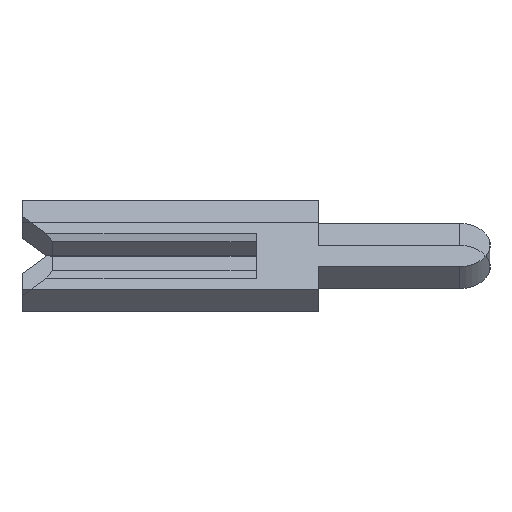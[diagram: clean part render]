
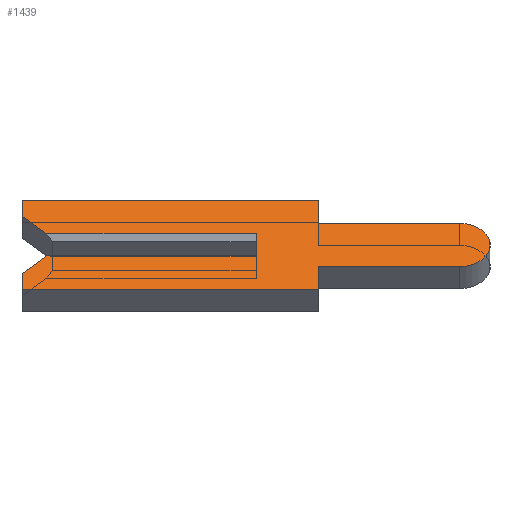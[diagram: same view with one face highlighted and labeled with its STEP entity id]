
A CAD part, left-side view. The second image highlights one B-rep face of the part: STEP entity #1439.
In plain terms, the highlighted face is planar.
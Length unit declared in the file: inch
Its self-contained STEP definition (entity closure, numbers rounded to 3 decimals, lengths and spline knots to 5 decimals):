
#7 = DIRECTION ( 'NONE',  ( 0., -1., 0. ) ) ;
#17 = DIRECTION ( 'NONE',  ( 0., 0., -1. ) ) ;
#46 = VERTEX_POINT ( 'NONE', #1941 ) ;
#65 = LINE ( 'NONE', #826, #1199 ) ;
#94 = VERTEX_POINT ( 'NONE', #2145 ) ;
#114 = EDGE_CURVE ( 'NONE', #2281, #2518, #854, .T. ) ;
#122 = CARTESIAN_POINT ( 'NONE',  ( -0.01, -0.04, 0.0195 ) ) ;
#156 = CARTESIAN_POINT ( 'NONE',  ( -0.01, 0.15, 0.026 ) ) ;
#189 = CARTESIAN_POINT ( 'NONE',  ( -0.01, -0.1305, 0.0195 ) ) ;
#202 = VERTEX_POINT ( 'NONE', #189 ) ;
#210 = VECTOR ( 'NONE', #1328, 39.37008 ) ;
#230 = EDGE_CURVE ( 'NONE', #1036, #2063, #1580, .T. ) ;
#243 = LINE ( 'NONE', #156, #2073 ) ;
#271 = EDGE_CURVE ( 'NONE', #1648, #94, #506, .T. ) ;
#272 = VECTOR ( 'NONE', #17, 39.37008 ) ;
#276 = VECTOR ( 'NONE', #582, 39.37008 ) ;
#277 = LINE ( 'NONE', #926, #210 ) ;
#283 = CARTESIAN_POINT ( 'NONE',  ( -0.01, 0.134, 0.01 ) ) ;
#305 = PLANE ( 'NONE',  #306 ) ;
#306 = AXIS2_PLACEMENT_3D ( 'NONE', #1707, #718, #921 ) ;
#350 = CARTESIAN_POINT ( 'NONE',  ( -0.01, 0.15, -0.04 ) ) ;
#405 = FACE_OUTER_BOUND ( 'NONE', #1035, .T. ) ;
#424 = EDGE_CURVE ( 'NONE', #1326, #1935, #1843, .T. ) ;
#500 = VECTOR ( 'NONE', #2418, 39.37008 ) ;
#506 = LINE ( 'NONE', #614, #1052 ) ;
#560 = VECTOR ( 'NONE', #1524, 39.37008 ) ;
#563 = DIRECTION ( 'NONE',  ( 0., 1., 0. ) ) ;
#579 = CARTESIAN_POINT ( 'NONE',  ( -0.01, 0.134, -0.01 ) ) ;
#582 = DIRECTION ( 'NONE',  ( 0., -0.707, 0.707 ) ) ;
#612 = VERTEX_POINT ( 'NONE', #2058 ) ;
#614 = CARTESIAN_POINT ( 'NONE',  ( -0.01, 0.15, 0.04 ) ) ;
#648 = EDGE_CURVE ( 'NONE', #202, #1647, #860, .T. ) ;
#718 = DIRECTION ( 'NONE',  ( 1., 0., 0. ) ) ;
#787 = VECTOR ( 'NONE', #2552, 39.37008 ) ;
#804 = CARTESIAN_POINT ( 'NONE',  ( -0.01, 0.1305, 0.0065 ) ) ;
#819 = VECTOR ( 'NONE', #1531, 39.37008 ) ;
#826 = CARTESIAN_POINT ( 'NONE',  ( -0.01, 0.15, 0.01 ) ) ;
#829 = ORIENTED_EDGE ( 'NONE', *, *, #1122, .F. ) ;
#854 = LINE ( 'NONE', #1562, #276 ) ;
#860 = CIRCLE ( 'NONE', #1827, 0.0195 ) ;
#907 = ORIENTED_EDGE ( 'NONE', *, *, #2233, .F. ) ;
#910 = CARTESIAN_POINT ( 'NONE',  ( -0.01, -0.04, -0.0195 ) ) ;
#921 = DIRECTION ( 'NONE',  ( 0., 0., -1. ) ) ;
#926 = CARTESIAN_POINT ( 'NONE',  ( -0.01, 0.15, -0.026 ) ) ;
#945 = LINE ( 'NONE', #1614, #1886 ) ;
#969 = CARTESIAN_POINT ( 'NONE',  ( -0.01, 0.15, 0.04 ) ) ;
#1035 = EDGE_LOOP ( 'NONE', ( #1040, #829, #907, #2174, #1686, #1324, #2101, #2035, #1656, #2122, #1872, #2027, #1849, #1943 ) ) ;
#1036 = VERTEX_POINT ( 'NONE', #283 ) ;
#1040 = ORIENTED_EDGE ( 'NONE', *, *, #2375, .T. ) ;
#1052 = VECTOR ( 'NONE', #1826, 39.37008 ) ;
#1113 = CARTESIAN_POINT ( 'NONE',  ( -0.01, 0., 0.0065 ) ) ;
#1122 = EDGE_CURVE ( 'NONE', #2093, #46, #1205, .T. ) ;
#1175 = EDGE_CURVE ( 'NONE', #612, #202, #1953, .T. ) ;
#1193 = EDGE_CURVE ( 'NONE', #1728, #2281, #277, .T. ) ;
#1199 = VECTOR ( 'NONE', #7, 39.37008 ) ;
#1205 = LINE ( 'NONE', #1113, #787 ) ;
#1277 = VECTOR ( 'NONE', #563, 39.37008 ) ;
#1319 = CARTESIAN_POINT ( 'NONE',  ( -0.01, -0.1305, 0. ) ) ;
#1324 = ORIENTED_EDGE ( 'NONE', *, *, #2412, .F. ) ;
#1326 = VERTEX_POINT ( 'NONE', #910 ) ;
#1328 = DIRECTION ( 'NONE',  ( 0., 0., 1. ) ) ;
#1382 = EDGE_CURVE ( 'NONE', #94, #612, #2306, .T. ) ;
#1439 = ADVANCED_FACE ( 'NONE', ( #405 ), #305, .F. ) ;
#1490 = LINE ( 'NONE', #2156, #1277 ) ;
#1524 = DIRECTION ( 'NONE',  ( 0., 0., -1. ) ) ;
#1531 = DIRECTION ( 'NONE',  ( 0., -1., 0. ) ) ;
#1562 = CARTESIAN_POINT ( 'NONE',  ( -0.01, 0.1305, -0.0065 ) ) ;
#1566 = CARTESIAN_POINT ( 'NONE',  ( -0.01, 0.15, 0.026 ) ) ;
#1580 = LINE ( 'NONE', #804, #500 ) ;
#1614 = CARTESIAN_POINT ( 'NONE',  ( -0.01, -0.1305, -0.01 ) ) ;
#1647 = VERTEX_POINT ( 'NONE', #1755 ) ;
#1648 = VERTEX_POINT ( 'NONE', #969 ) ;
#1656 = ORIENTED_EDGE ( 'NONE', *, *, #648, .F. ) ;
#1667 = DIRECTION ( 'NONE',  ( 0., 0., -1. ) ) ;
#1686 = ORIENTED_EDGE ( 'NONE', *, *, #1193, .F. ) ;
#1707 = CARTESIAN_POINT ( 'NONE',  ( -0.01, -0.1305, 0. ) ) ;
#1710 = CARTESIAN_POINT ( 'NONE',  ( -0.01, -0.04, 0.04 ) ) ;
#1728 = VERTEX_POINT ( 'NONE', #350 ) ;
#1735 = DIRECTION ( 'NONE',  ( 0., 0., 1. ) ) ;
#1755 = CARTESIAN_POINT ( 'NONE',  ( -0.01, -0.1305, -0.0195 ) ) ;
#1777 = DIRECTION ( 'NONE',  ( 0., -1., 0. ) ) ;
#1784 = DIRECTION ( 'NONE',  ( 0., 1., 0. ) ) ;
#1826 = DIRECTION ( 'NONE',  ( 0., -1., 0. ) ) ;
#1827 = AXIS2_PLACEMENT_3D ( 'NONE', #1319, #2272, #1667 ) ;
#1843 = LINE ( 'NONE', #2219, #272 ) ;
#1849 = ORIENTED_EDGE ( 'NONE', *, *, #1997, .F. ) ;
#1872 = ORIENTED_EDGE ( 'NONE', *, *, #1382, .F. ) ;
#1886 = VECTOR ( 'NONE', #1777, 39.37008 ) ;
#1935 = VERTEX_POINT ( 'NONE', #2382 ) ;
#1941 = CARTESIAN_POINT ( 'NONE',  ( -0.01, 0., 0.01 ) ) ;
#1943 = ORIENTED_EDGE ( 'NONE', *, *, #230, .F. ) ;
#1953 = LINE ( 'NONE', #122, #819 ) ;
#1997 = EDGE_CURVE ( 'NONE', #2063, #1648, #243, .T. ) ;
#2008 = LINE ( 'NONE', #2407, #2333 ) ;
#2027 = ORIENTED_EDGE ( 'NONE', *, *, #271, .F. ) ;
#2035 = ORIENTED_EDGE ( 'NONE', *, *, #2079, .F. ) ;
#2058 = CARTESIAN_POINT ( 'NONE',  ( -0.01, -0.04, 0.0195 ) ) ;
#2063 = VERTEX_POINT ( 'NONE', #1566 ) ;
#2073 = VECTOR ( 'NONE', #1735, 39.37008 ) ;
#2079 = EDGE_CURVE ( 'NONE', #1647, #1326, #1490, .T. ) ;
#2093 = VERTEX_POINT ( 'NONE', #2152 ) ;
#2101 = ORIENTED_EDGE ( 'NONE', *, *, #424, .F. ) ;
#2122 = ORIENTED_EDGE ( 'NONE', *, *, #1175, .F. ) ;
#2145 = CARTESIAN_POINT ( 'NONE',  ( -0.01, -0.04, 0.04 ) ) ;
#2152 = CARTESIAN_POINT ( 'NONE',  ( -0.01, 0., -0.01 ) ) ;
#2156 = CARTESIAN_POINT ( 'NONE',  ( -0.01, -0.04, -0.0195 ) ) ;
#2174 = ORIENTED_EDGE ( 'NONE', *, *, #114, .F. ) ;
#2198 = CARTESIAN_POINT ( 'NONE',  ( -0.01, 0.15, -0.026 ) ) ;
#2219 = CARTESIAN_POINT ( 'NONE',  ( -0.01, -0.04, -0.04 ) ) ;
#2233 = EDGE_CURVE ( 'NONE', #2518, #2093, #945, .T. ) ;
#2272 = DIRECTION ( 'NONE',  ( 1., 0., 0. ) ) ;
#2281 = VERTEX_POINT ( 'NONE', #2198 ) ;
#2306 = LINE ( 'NONE', #1710, #560 ) ;
#2333 = VECTOR ( 'NONE', #1784, 39.37008 ) ;
#2375 = EDGE_CURVE ( 'NONE', #1036, #46, #65, .T. ) ;
#2382 = CARTESIAN_POINT ( 'NONE',  ( -0.01, -0.04, -0.04 ) ) ;
#2407 = CARTESIAN_POINT ( 'NONE',  ( -0.01, 0.15, -0.04 ) ) ;
#2412 = EDGE_CURVE ( 'NONE', #1935, #1728, #2008, .T. ) ;
#2418 = DIRECTION ( 'NONE',  ( 0., 0.707, 0.707 ) ) ;
#2518 = VERTEX_POINT ( 'NONE', #579 ) ;
#2552 = DIRECTION ( 'NONE',  ( 0., 0., 1. ) ) ;
